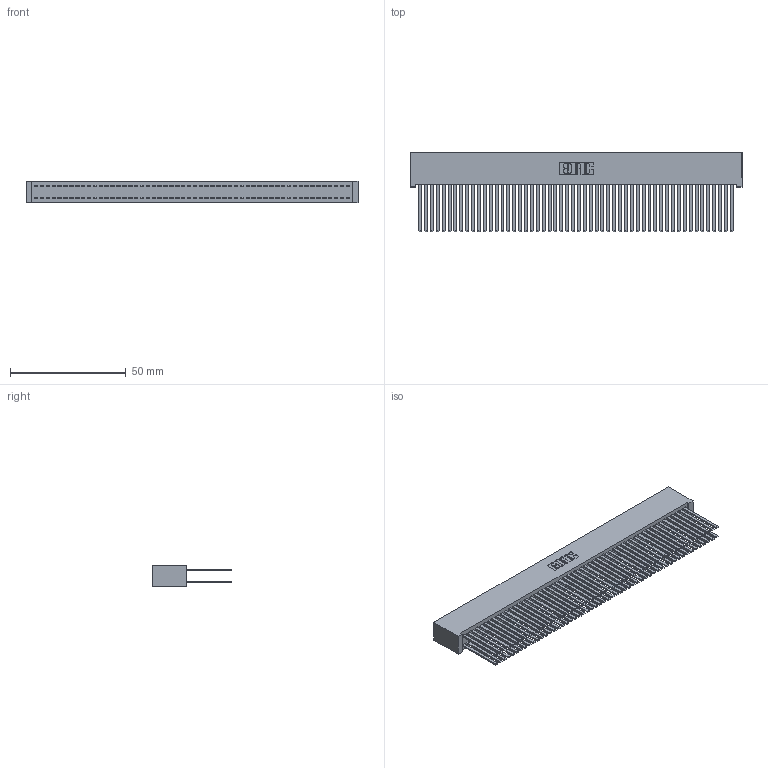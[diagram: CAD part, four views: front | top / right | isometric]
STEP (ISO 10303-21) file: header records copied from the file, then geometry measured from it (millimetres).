
FILE_DESCRIPTION (( 'STEP AP203' ), '1' );
FILE_NAME ('392-108-544-201.STEP', '2019-10-09T23:14:36', ( '' ), ( '' ), 'SwSTEP 2.0', 'SolidWorks 2016', '' );
FILE_SCHEMA (( 'CONFIG_CONTROL_DESIGN' ));
Length unit declared in the file: inch
Products named in the file (3): 342 Part_Lugless; 345-292-001_345-293-144; 392-108-544-201
Assembly tree (109 placements, depth 2):
  392-108-544-201
    342 Part_Lugless
    345-292-001_345-293-144  x108
Bounding box: 143.41 x 34.3 x 9.4 mm (x, y, z)
Volume: 14895.5 mm3; surface area: 29180.7 mm2
Topology: 109 solids, 109 shells, 5070 faces, 15071 edges, 9902 vertices
Faces by surface type: plane 3518, cylinder 1552
Entity records: 32595 total; most frequent: CARTESIAN_POINT 5382, ORIENTED_EDGE 5318, DIRECTION 4567, EDGE_CURVE 2659, VECTOR 2543, LINE 2543, VERTEX_POINT 1770, AXIS2_PLACEMENT_3D 1012
